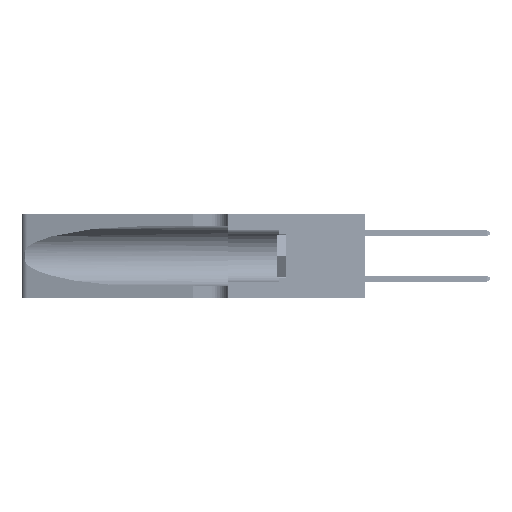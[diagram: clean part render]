
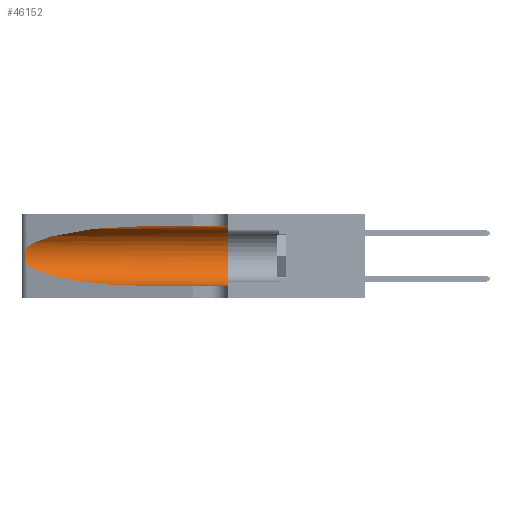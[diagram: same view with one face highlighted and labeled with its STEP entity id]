
A CAD part, left-side view. The second image highlights one B-rep face of the part: STEP entity #46152.
In plain terms, the highlighted cylindrical face has radius 3.308 mm (diameter 6.617 mm), a partial arc.
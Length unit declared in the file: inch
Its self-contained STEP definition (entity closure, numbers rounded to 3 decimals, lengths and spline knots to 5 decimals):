
#2573 =( BOUNDED_CURVE ( )  B_SPLINE_CURVE ( 3, ( #18466, #33531, #37957, #10455 ),
 .UNSPECIFIED., .F., .T. ) 
 B_SPLINE_CURVE_WITH_KNOTS ( ( 4, 4 ),
 ( 1.5708, 2.84003 ),
 .UNSPECIFIED. ) 
 CURVE ( )  GEOMETRIC_REPRESENTATION_ITEM ( )  RATIONAL_B_SPLINE_CURVE ( ( 1., 0.87, 0.87, 1. ) ) 
 REPRESENTATION_ITEM ( '' )  );
#4012 = FACE_OUTER_BOUND ( 'NONE', #14458, .T. ) ;
#4265 = EDGE_CURVE ( 'NONE', #37113, #18473, #39603, .T. ) ;
#5274 = CARTESIAN_POINT ( 'NONE',  ( 0.2373, 1.15595, 0.08982 ) ) ;
#6300 = CARTESIAN_POINT ( 'NONE',  ( 0.26075, 1.23896, 0.19203 ) ) ;
#6464 = CARTESIAN_POINT ( 'NONE',  ( 0.25787, 1.23484, 0.2124 ) ) ;
#6630 = CARTESIAN_POINT ( 'NONE',  ( 0.25639, 1.23184, 0.21858 ) ) ;
#6668 = DIRECTION ( 'NONE',  ( 0., -1., 0. ) ) ;
#7239 = DIRECTION ( 'NONE',  ( 0., -1., 0. ) ) ;
#7511 = VERTEX_POINT ( 'NONE', #34428 ) ;
#9156 = ORIENTED_EDGE ( 'NONE', *, *, #14873, .T. ) ;
#9203 = CARTESIAN_POINT ( 'NONE',  ( 0.1305, 0.72297, 0.05475 ) ) ;
#10455 = CARTESIAN_POINT ( 'NONE',  ( 0.25487, 1.22718, 0.22369 ) ) ;
#10566 = CARTESIAN_POINT ( 'NONE',  ( 0.25639, 1.23186, 0.15144 ) ) ;
#10766 = B_SPLINE_CURVE_WITH_KNOTS ( 'NONE', 3,
 ( #30066, #33631, #6630, #6464, #25794, #29752, #6300, #18081, #37572, #14354, #33966, #10566, #37896, #41893 ),
 .UNSPECIFIED., .F., .F.,
 ( 4, 2, 2, 2, 2, 2, 4 ),
 ( 0., 0.00027, 0.00053, 0.00107, 0.0016, 0.00187, 0.00214 ),
 .UNSPECIFIED. ) ;
#11770 = VERTEX_POINT ( 'NONE', #38987 ) ;
#14354 = CARTESIAN_POINT ( 'NONE',  ( 0.25856, 1.23593, 0.16098 ) ) ;
#14458 = EDGE_LOOP ( 'NONE', ( #21647, #33912, #9156, #49861, #36943, #26094 ) ) ;
#14789 = CARTESIAN_POINT ( 'NONE',  ( 0.1305, 0.72297, 0.31525 ) ) ;
#14873 = EDGE_CURVE ( 'NONE', #34829, #41208, #34239, .T. ) ;
#17214 = CARTESIAN_POINT ( 'NONE',  ( 0.1305, 0.72297, 0.05475 ) ) ;
#18079 = VECTOR ( 'NONE', #25651, 39.37008 ) ;
#18081 = CARTESIAN_POINT ( 'NONE',  ( 0.26075, 1.23896, 0.178 ) ) ;
#18466 = CARTESIAN_POINT ( 'NONE',  ( 0.1305, 0.72297, 0.31525 ) ) ;
#18473 = VERTEX_POINT ( 'NONE', #19030 ) ;
#18812 = AXIS2_PLACEMENT_3D ( 'NONE', #50425, #37496, #45428 ) ;
#19030 = CARTESIAN_POINT ( 'NONE',  ( 0.1305, 0.35, 0.31525 ) ) ;
#21647 = ORIENTED_EDGE ( 'NONE', *, *, #43004, .T. ) ;
#22401 = CARTESIAN_POINT ( 'NONE',  ( 0.1305, 1.61858, 0.05475 ) ) ;
#22934 = EDGE_CURVE ( 'NONE', #41208, #7511, #36445, .T. ) ;
#24322 = CIRCLE ( 'NONE', #18812, 0.13025 ) ;
#25651 = DIRECTION ( 'NONE',  ( 0., -1., 0. ) ) ;
#25794 = CARTESIAN_POINT ( 'NONE',  ( 0.25854, 1.2359, 0.20912 ) ) ;
#26094 = ORIENTED_EDGE ( 'NONE', *, *, #4265, .F. ) ;
#29752 = CARTESIAN_POINT ( 'NONE',  ( 0.26018, 1.23835, 0.19895 ) ) ;
#30066 = CARTESIAN_POINT ( 'NONE',  ( 0.25487, 1.22718, 0.22369 ) ) ;
#30113 = CARTESIAN_POINT ( 'NONE',  ( 0.1305, 1.61858, 0.185 ) ) ;
#32604 = CARTESIAN_POINT ( 'NONE',  ( 0.18966, 0.96281, 0.05475 ) ) ;
#33212 = EDGE_CURVE ( 'NONE', #18473, #7511, #24322, .T. ) ;
#33531 = CARTESIAN_POINT ( 'NONE',  ( 0.18966, 0.96281, 0.31525 ) ) ;
#33631 = CARTESIAN_POINT ( 'NONE',  ( 0.25555, 1.22994, 0.2215 ) ) ;
#33912 = ORIENTED_EDGE ( 'NONE', *, *, #43743, .T. ) ;
#33966 = CARTESIAN_POINT ( 'NONE',  ( 0.25789, 1.23486, 0.15765 ) ) ;
#34013 = DIRECTION ( 'NONE',  ( 0., 0., -1. ) ) ;
#34220 = CARTESIAN_POINT ( 'NONE',  ( 0.1305, 1.61858, 0.31525 ) ) ;
#34239 =( BOUNDED_CURVE ( )  B_SPLINE_CURVE ( 3, ( #44304, #5274, #32604, #9203 ),
 .UNSPECIFIED., .F., .F. ) 
 B_SPLINE_CURVE_WITH_KNOTS ( ( 4, 4 ),
 ( 3.44316, 4.71239 ),
 .UNSPECIFIED. ) 
 CURVE ( )  GEOMETRIC_REPRESENTATION_ITEM ( )  RATIONAL_B_SPLINE_CURVE ( ( 1., 0.87, 0.87, 1. ) ) 
 REPRESENTATION_ITEM ( '' )  );
#34428 = CARTESIAN_POINT ( 'NONE',  ( 0.1305, 0.35, 0.05475 ) ) ;
#34829 = VERTEX_POINT ( 'NONE', #35678 ) ;
#35678 = CARTESIAN_POINT ( 'NONE',  ( 0.25487, 1.22718, 0.14631 ) ) ;
#36445 = LINE ( 'NONE', #22401, #18079 ) ;
#36943 = ORIENTED_EDGE ( 'NONE', *, *, #33212, .F. ) ;
#37113 = VERTEX_POINT ( 'NONE', #14789 ) ;
#37496 = DIRECTION ( 'NONE',  ( 0., 1., 0. ) ) ;
#37572 = CARTESIAN_POINT ( 'NONE',  ( 0.26017, 1.23833, 0.17102 ) ) ;
#37896 = CARTESIAN_POINT ( 'NONE',  ( 0.25555, 1.22993, 0.14849 ) ) ;
#37957 = CARTESIAN_POINT ( 'NONE',  ( 0.2373, 1.15595, 0.28018 ) ) ;
#38987 = CARTESIAN_POINT ( 'NONE',  ( 0.25487, 1.22718, 0.22369 ) ) ;
#39603 = LINE ( 'NONE', #34220, #46370 ) ;
#41208 = VERTEX_POINT ( 'NONE', #17214 ) ;
#41893 = CARTESIAN_POINT ( 'NONE',  ( 0.25487, 1.22718, 0.14631 ) ) ;
#43004 = EDGE_CURVE ( 'NONE', #37113, #11770, #2573, .T. ) ;
#43743 = EDGE_CURVE ( 'NONE', #11770, #34829, #10766, .T. ) ;
#44304 = CARTESIAN_POINT ( 'NONE',  ( 0.25487, 1.22718, 0.14631 ) ) ;
#45124 = AXIS2_PLACEMENT_3D ( 'NONE', #30113, #6668, #34013 ) ;
#45428 = DIRECTION ( 'NONE',  ( 0., 0., 1. ) ) ;
#45690 = CYLINDRICAL_SURFACE ( 'NONE', #45124, 0.13025 ) ;
#46152 = ADVANCED_FACE ( 'NONE', ( #4012 ), #45690, .F. ) ;
#46370 = VECTOR ( 'NONE', #7239, 39.37008 ) ;
#49861 = ORIENTED_EDGE ( 'NONE', *, *, #22934, .T. ) ;
#50425 = CARTESIAN_POINT ( 'NONE',  ( 0.1305, 0.35, 0.185 ) ) ;
